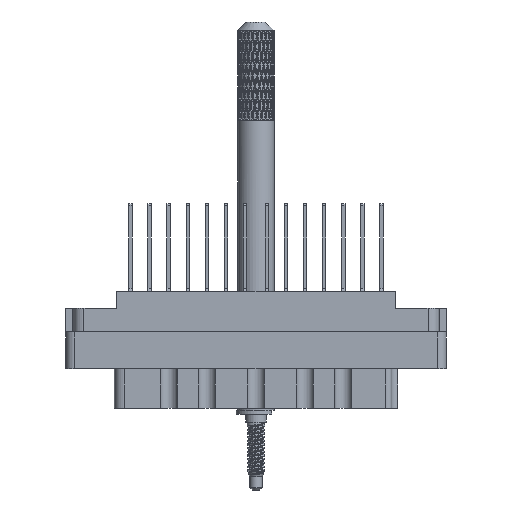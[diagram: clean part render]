
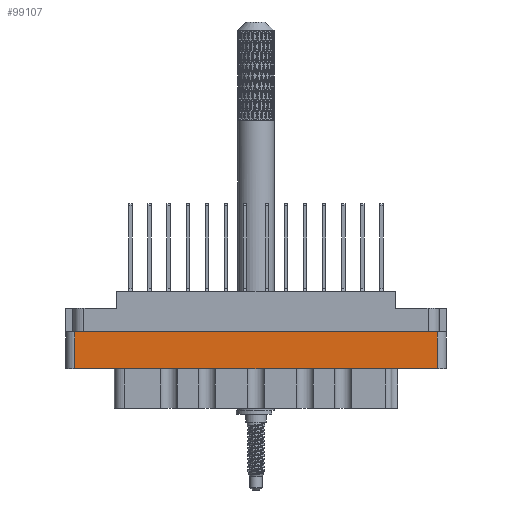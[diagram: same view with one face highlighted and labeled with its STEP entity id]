
A CAD part, front view. The second image highlights one B-rep face of the part: STEP entity #99107.
In plain terms, the highlighted planar face has unit normal (0, -1, 0).
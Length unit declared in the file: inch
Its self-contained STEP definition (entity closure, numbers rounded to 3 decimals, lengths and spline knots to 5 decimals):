
#162 = VECTOR ( 'NONE', #89838, 39.37008 ) ;
#2339 = CARTESIAN_POINT ( 'NONE',  ( 1.234, -0.438, -0.277 ) ) ;
#7159 = CARTESIAN_POINT ( 'NONE',  ( -1.296, -0.438, -0.798 ) ) ;
#7768 = VERTEX_POINT ( 'NONE', #2339 ) ;
#8124 = VERTEX_POINT ( 'NONE', #34960 ) ;
#9618 = ORIENTED_EDGE ( 'NONE', *, *, #41644, .T. ) ;
#9967 = ORIENTED_EDGE ( 'NONE', *, *, #29319, .T. ) ;
#16161 = EDGE_CURVE ( 'NONE', #78263, #7768, #68525, .T. ) ;
#18583 = LINE ( 'NONE', #98090, #50979 ) ;
#27633 = EDGE_CURVE ( 'NONE', #8124, #32670, #41269, .T. ) ;
#29319 = EDGE_CURVE ( 'NONE', #78263, #32670, #18583, .T. ) ;
#30446 = CARTESIAN_POINT ( 'NONE',  ( 0., -0.438, -0.277 ) ) ;
#32670 = VERTEX_POINT ( 'NONE', #77425 ) ;
#34960 = CARTESIAN_POINT ( 'NONE',  ( 1.234, -0.438, -0.529 ) ) ;
#38859 = DIRECTION ( 'NONE',  ( -1., 0., 0. ) ) ;
#39886 = ORIENTED_EDGE ( 'NONE', *, *, #27633, .F. ) ;
#41269 = LINE ( 'NONE', #84275, #66693 ) ;
#41644 = EDGE_CURVE ( 'NONE', #8124, #7768, #80667, .T. ) ;
#50979 = VECTOR ( 'NONE', #62060, 39.37008 ) ;
#51970 = FACE_OUTER_BOUND ( 'NONE', #85655, .T. ) ;
#54969 = ORIENTED_EDGE ( 'NONE', *, *, #16161, .F. ) ;
#62060 = DIRECTION ( 'NONE',  ( 0., 0., -1. ) ) ;
#66693 = VECTOR ( 'NONE', #38859, 39.37008 ) ;
#66730 = DIRECTION ( 'NONE',  ( 1., 0., 0. ) ) ;
#68525 = LINE ( 'NONE', #30446, #101095 ) ;
#70201 = DIRECTION ( 'NONE',  ( 0., 0., -1. ) ) ;
#70319 = CARTESIAN_POINT ( 'NONE',  ( -1.234, -0.438, -0.277 ) ) ;
#77425 = CARTESIAN_POINT ( 'NONE',  ( -1.234, -0.438, -0.529 ) ) ;
#78263 = VERTEX_POINT ( 'NONE', #70319 ) ;
#80667 = LINE ( 'NONE', #100936, #162 ) ;
#84275 = CARTESIAN_POINT ( 'NONE',  ( 0., -0.438, -0.529 ) ) ;
#85655 = EDGE_LOOP ( 'NONE', ( #54969, #9967, #39886, #9618 ) ) ;
#88785 = DIRECTION ( 'NONE',  ( 0., -1., 0. ) ) ;
#89838 = DIRECTION ( 'NONE',  ( 0., 0., 1. ) ) ;
#97898 = PLANE ( 'NONE',  #99634 ) ;
#98090 = CARTESIAN_POINT ( 'NONE',  ( -1.234, -0.438, -0.798 ) ) ;
#99107 = ADVANCED_FACE ( 'NONE', ( #51970 ), #97898, .T. ) ;
#99634 = AXIS2_PLACEMENT_3D ( 'NONE', #7159, #88785, #70201 ) ;
#100936 = CARTESIAN_POINT ( 'NONE',  ( 1.234, -0.438, -0.798 ) ) ;
#101095 = VECTOR ( 'NONE', #66730, 39.37008 ) ;
